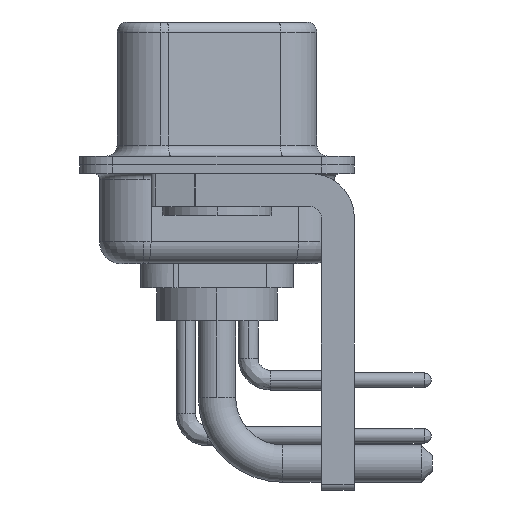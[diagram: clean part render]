
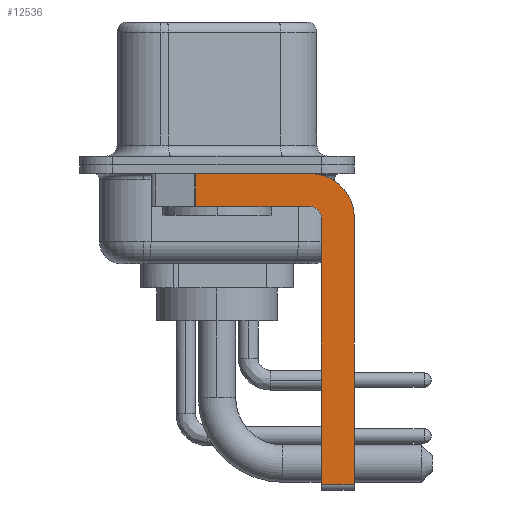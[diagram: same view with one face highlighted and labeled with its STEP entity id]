
A CAD part, left-side view. The second image highlights one B-rep face of the part: STEP entity #12536.
In plain terms, the highlighted planar face has unit normal (-1, 0, 0).
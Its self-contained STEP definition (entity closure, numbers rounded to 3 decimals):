
#155 = DIRECTION ( 'NONE',  ( -1., 0., 0. ) ) ;
#174 = EDGE_CURVE ( 'NONE', #16372, #15336, #16317, .T. ) ;
#411 = DIRECTION ( 'NONE',  ( 0., 0., -1. ) ) ;
#551 = EDGE_CURVE ( 'NONE', #3760, #15336, #7089, .T. ) ;
#1402 = LINE ( 'NONE', #2410, #2500 ) ;
#1419 = AXIS2_PLACEMENT_3D ( 'NONE', #10205, #155, #6542 ) ;
#1661 = EDGE_LOOP ( 'NONE', ( #18871, #26034, #3688, #11022, #10450, #4696, #12515, #5388 ) ) ;
#2149 = CARTESIAN_POINT ( 'NONE',  ( -2.9, 0.978, -0.4 ) ) ;
#2410 = CARTESIAN_POINT ( 'NONE',  ( -2.9, -4.75, -14.8 ) ) ;
#2500 = VECTOR ( 'NONE', #22138, 1000. ) ;
#3000 = VERTEX_POINT ( 'NONE', #6563 ) ;
#3529 = VECTOR ( 'NONE', #5847, 1000. ) ;
#3599 = DIRECTION ( 'NONE',  ( 0., 0., -1. ) ) ;
#3688 = ORIENTED_EDGE ( 'NONE', *, *, #7442, .F. ) ;
#3760 = VERTEX_POINT ( 'NONE', #11364 ) ;
#4696 = ORIENTED_EDGE ( 'NONE', *, *, #551, .T. ) ;
#4981 = EDGE_CURVE ( 'NONE', #3760, #3000, #1402, .T. ) ;
#5388 = ORIENTED_EDGE ( 'NONE', *, *, #21289, .F. ) ;
#5627 = CARTESIAN_POINT ( 'NONE',  ( -2.9, -4.25, -2.4 ) ) ;
#5847 = DIRECTION ( 'NONE',  ( 0., -1., 0. ) ) ;
#6445 = VERTEX_POINT ( 'NONE', #26742 ) ;
#6484 = LINE ( 'NONE', #19831, #27888 ) ;
#6542 = DIRECTION ( 'NONE',  ( 0., 0., 1. ) ) ;
#6563 = CARTESIAN_POINT ( 'NONE',  ( -2.9, -4.75, -2.4 ) ) ;
#6815 = DIRECTION ( 'NONE',  ( 0., -1., 0. ) ) ;
#7089 = LINE ( 'NONE', #15915, #23362 ) ;
#7442 = EDGE_CURVE ( 'NONE', #15825, #10048, #11955, .T. ) ;
#9004 = EDGE_CURVE ( 'NONE', #13961, #10048, #6484, .T. ) ;
#9691 = PLANE ( 'NONE',  #18213 ) ;
#10048 = VERTEX_POINT ( 'NONE', #27687 ) ;
#10205 = CARTESIAN_POINT ( 'NONE',  ( -2.9, -4.25, -2.4 ) ) ;
#10450 = ORIENTED_EDGE ( 'NONE', *, *, #4981, .F. ) ;
#11022 = ORIENTED_EDGE ( 'NONE', *, *, #27331, .F. ) ;
#11315 = DIRECTION ( 'NONE',  ( 1., 0., 0. ) ) ;
#11364 = CARTESIAN_POINT ( 'NONE',  ( -2.9, -4.75, -14.55 ) ) ;
#11932 = LINE ( 'NONE', #16994, #3529 ) ;
#11955 = LINE ( 'NONE', #27488, #18984 ) ;
#12515 = ORIENTED_EDGE ( 'NONE', *, *, #174, .F. ) ;
#12536 = ADVANCED_FACE ( 'NONE', ( #23185 ), #9691, .F. ) ;
#13467 = CARTESIAN_POINT ( 'NONE',  ( -2.9, -4.25, -1.9 ) ) ;
#13961 = VERTEX_POINT ( 'NONE', #2149 ) ;
#14936 = EDGE_CURVE ( 'NONE', #13961, #6445, #11932, .T. ) ;
#15336 = VERTEX_POINT ( 'NONE', #27157 ) ;
#15825 = VERTEX_POINT ( 'NONE', #13467 ) ;
#15915 = CARTESIAN_POINT ( 'NONE',  ( -2.9, -4.25, -14.55 ) ) ;
#16131 = CARTESIAN_POINT ( 'NONE',  ( -2.9, -6.25, -2.4 ) ) ;
#16317 = LINE ( 'NONE', #20283, #27524 ) ;
#16372 = VERTEX_POINT ( 'NONE', #16131 ) ;
#16464 = CIRCLE ( 'NONE', #27619, 2. ) ;
#16994 = CARTESIAN_POINT ( 'NONE',  ( -2.9, 3., -0.4 ) ) ;
#17992 = DIRECTION ( 'NONE',  ( 0., 0., -1. ) ) ;
#18213 = AXIS2_PLACEMENT_3D ( 'NONE', #5627, #21301, #3599 ) ;
#18871 = ORIENTED_EDGE ( 'NONE', *, *, #14936, .F. ) ;
#18984 = VECTOR ( 'NONE', #25760, 1000. ) ;
#19767 = CARTESIAN_POINT ( 'NONE',  ( -2.9, -4.25, -2.4 ) ) ;
#19831 = CARTESIAN_POINT ( 'NONE',  ( -2.9, 0.978, -1.9 ) ) ;
#19975 = DIRECTION ( 'NONE',  ( 0., 0., -1. ) ) ;
#20283 = CARTESIAN_POINT ( 'NONE',  ( -2.9, -6.25, -2.4 ) ) ;
#21289 = EDGE_CURVE ( 'NONE', #6445, #16372, #16464, .T. ) ;
#21301 = DIRECTION ( 'NONE',  ( 1., 0., 0. ) ) ;
#22138 = DIRECTION ( 'NONE',  ( 0., 0., 1. ) ) ;
#22275 = CIRCLE ( 'NONE', #1419, 0.5 ) ;
#23185 = FACE_OUTER_BOUND ( 'NONE', #1661, .T. ) ;
#23362 = VECTOR ( 'NONE', #6815, 1000. ) ;
#25760 = DIRECTION ( 'NONE',  ( 0., 1., 0. ) ) ;
#26034 = ORIENTED_EDGE ( 'NONE', *, *, #9004, .T. ) ;
#26742 = CARTESIAN_POINT ( 'NONE',  ( -2.9, -4.25, -0.4 ) ) ;
#27157 = CARTESIAN_POINT ( 'NONE',  ( -2.9, -6.25, -14.55 ) ) ;
#27331 = EDGE_CURVE ( 'NONE', #3000, #15825, #22275, .T. ) ;
#27488 = CARTESIAN_POINT ( 'NONE',  ( -2.9, -4.25, -1.9 ) ) ;
#27524 = VECTOR ( 'NONE', #411, 1000. ) ;
#27619 = AXIS2_PLACEMENT_3D ( 'NONE', #19767, #11315, #17992 ) ;
#27687 = CARTESIAN_POINT ( 'NONE',  ( -2.9, 0.978, -1.9 ) ) ;
#27888 = VECTOR ( 'NONE', #19975, 1000. ) ;
